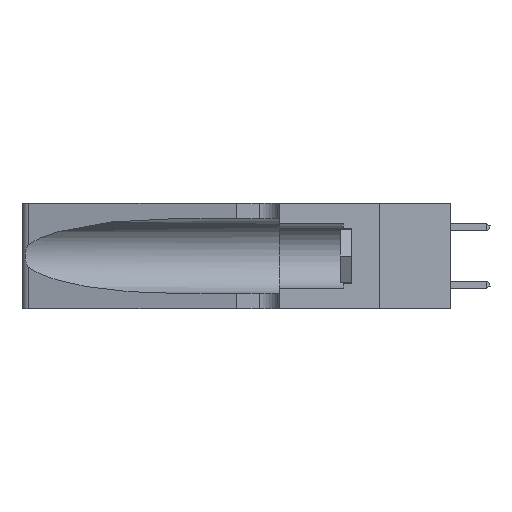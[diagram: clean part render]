
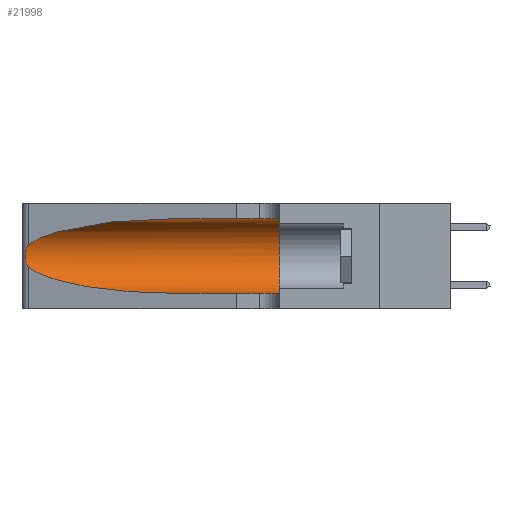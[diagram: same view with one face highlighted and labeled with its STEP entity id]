
A CAD part, left-side view. The second image highlights one B-rep face of the part: STEP entity #21998.
In plain terms, the highlighted cylindrical face has radius 3.308 mm (diameter 6.617 mm), a partial arc.
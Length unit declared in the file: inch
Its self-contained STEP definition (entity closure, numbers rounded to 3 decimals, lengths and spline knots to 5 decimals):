
#524 = CARTESIAN_POINT ( 'NONE',  ( 0.25487, 1.22718, 0.14631 ) ) ;
#641 = VERTEX_POINT ( 'NONE', #1984 ) ;
#919 = ORIENTED_EDGE ( 'NONE', *, *, #20815, .T. ) ;
#1160 = DIRECTION ( 'NONE',  ( 0., -1., 0. ) ) ;
#1449 = CYLINDRICAL_SURFACE ( 'NONE', #28516, 0.13025 ) ;
#1646 = VERTEX_POINT ( 'NONE', #9992 ) ;
#1953 = CARTESIAN_POINT ( 'NONE',  ( 0.25787, 1.23484, 0.2124 ) ) ;
#1984 = CARTESIAN_POINT ( 'NONE',  ( 0.1305, 0.72297, 0.31525 ) ) ;
#2099 = LINE ( 'NONE', #20987, #19862 ) ;
#2446 =( BOUNDED_CURVE ( )  B_SPLINE_CURVE ( 3, ( #29712, #20553, #8899, #18392 ),
 .UNSPECIFIED., .F., .F. ) 
 B_SPLINE_CURVE_WITH_KNOTS ( ( 4, 4 ),
 ( 1.5708, 2.84003 ),
 .UNSPECIFIED. ) 
 CURVE ( )  GEOMETRIC_REPRESENTATION_ITEM ( )  RATIONAL_B_SPLINE_CURVE ( ( 1., 0.87, 0.87, 1. ) ) 
 REPRESENTATION_ITEM ( '' )  );
#2768 = ORIENTED_EDGE ( 'NONE', *, *, #12227, .T. ) ;
#3309 = EDGE_CURVE ( 'NONE', #641, #1646, #25757, .T. ) ;
#3531 = CARTESIAN_POINT ( 'NONE',  ( 0.26075, 1.23896, 0.178 ) ) ;
#3865 = EDGE_CURVE ( 'NONE', #14556, #19030, #2099, .T. ) ;
#4131 = CARTESIAN_POINT ( 'NONE',  ( 0.25487, 1.22718, 0.14631 ) ) ;
#4221 = ORIENTED_EDGE ( 'NONE', *, *, #3309, .F. ) ;
#5302 = DIRECTION ( 'NONE',  ( 0., -1., 0. ) ) ;
#6467 = CARTESIAN_POINT ( 'NONE',  ( 0.25487, 1.22718, 0.14631 ) ) ;
#8374 = CARTESIAN_POINT ( 'NONE',  ( 0.25856, 1.23593, 0.16098 ) ) ;
#8885 = CARTESIAN_POINT ( 'NONE',  ( 0.25789, 1.23486, 0.15765 ) ) ;
#8899 = CARTESIAN_POINT ( 'NONE',  ( 0.2373, 1.15595, 0.28018 ) ) ;
#9102 = CARTESIAN_POINT ( 'NONE',  ( 0.26017, 1.23833, 0.17102 ) ) ;
#9992 = CARTESIAN_POINT ( 'NONE',  ( 0.1305, 0.35, 0.31525 ) ) ;
#10000 = CARTESIAN_POINT ( 'NONE',  ( 0.2373, 1.15595, 0.08982 ) ) ;
#10235 = B_SPLINE_CURVE_WITH_KNOTS ( 'NONE', 3,
 ( #23210, #20645, #24772, #1953, #27136, #25475, #23007, #3531, #9102, #8374, #8885, #20744, #20036, #4131 ),
 .UNSPECIFIED., .F., .F.,
 ( 4, 2, 2, 2, 2, 2, 4 ),
 ( 0., 0.00027, 0.00053, 0.00107, 0.0016, 0.00187, 0.00214 ),
 .UNSPECIFIED. ) ;
#11833 = ORIENTED_EDGE ( 'NONE', *, *, #3865, .T. ) ;
#12227 = EDGE_CURVE ( 'NONE', #22689, #14556, #13000, .T. ) ;
#13000 =( BOUNDED_CURVE ( )  B_SPLINE_CURVE ( 3, ( #524, #10000, #17386, #19578 ),
 .UNSPECIFIED., .F., .T. ) 
 B_SPLINE_CURVE_WITH_KNOTS ( ( 4, 4 ),
 ( 3.44316, 4.71239 ),
 .UNSPECIFIED. ) 
 CURVE ( )  GEOMETRIC_REPRESENTATION_ITEM ( )  RATIONAL_B_SPLINE_CURVE ( ( 1., 0.87, 0.87, 1. ) ) 
 REPRESENTATION_ITEM ( '' )  );
#13877 = EDGE_LOOP ( 'NONE', ( #28244, #919, #2768, #11833, #23106, #4221 ) ) ;
#14210 = EDGE_CURVE ( 'NONE', #641, #27275, #2446, .T. ) ;
#14556 = VERTEX_POINT ( 'NONE', #19638 ) ;
#15070 = CARTESIAN_POINT ( 'NONE',  ( 0.1305, 0.35, 0.185 ) ) ;
#15837 = CARTESIAN_POINT ( 'NONE',  ( 0.1305, 0.35, 0.05475 ) ) ;
#15981 = CARTESIAN_POINT ( 'NONE',  ( 0.25487, 1.22718, 0.22369 ) ) ;
#16174 = VECTOR ( 'NONE', #5302, 39.37008 ) ;
#16952 = CARTESIAN_POINT ( 'NONE',  ( 0.1305, 1.61858, 0.31525 ) ) ;
#17386 = CARTESIAN_POINT ( 'NONE',  ( 0.18966, 0.96281, 0.05475 ) ) ;
#17399 = DIRECTION ( 'NONE',  ( 0., 0., -1. ) ) ;
#17624 = AXIS2_PLACEMENT_3D ( 'NONE', #15070, #19726, #22057 ) ;
#18392 = CARTESIAN_POINT ( 'NONE',  ( 0.25487, 1.22718, 0.22369 ) ) ;
#19030 = VERTEX_POINT ( 'NONE', #15837 ) ;
#19578 = CARTESIAN_POINT ( 'NONE',  ( 0.1305, 0.72297, 0.05475 ) ) ;
#19638 = CARTESIAN_POINT ( 'NONE',  ( 0.1305, 0.72297, 0.05475 ) ) ;
#19726 = DIRECTION ( 'NONE',  ( 0., 1., 0. ) ) ;
#19862 = VECTOR ( 'NONE', #25723, 39.37008 ) ;
#19982 = CARTESIAN_POINT ( 'NONE',  ( 0.1305, 1.61858, 0.185 ) ) ;
#20036 = CARTESIAN_POINT ( 'NONE',  ( 0.25555, 1.22993, 0.14849 ) ) ;
#20319 = FACE_OUTER_BOUND ( 'NONE', #13877, .T. ) ;
#20553 = CARTESIAN_POINT ( 'NONE',  ( 0.18966, 0.96281, 0.31525 ) ) ;
#20645 = CARTESIAN_POINT ( 'NONE',  ( 0.25555, 1.22994, 0.2215 ) ) ;
#20744 = CARTESIAN_POINT ( 'NONE',  ( 0.25639, 1.23186, 0.15144 ) ) ;
#20815 = EDGE_CURVE ( 'NONE', #27275, #22689, #10235, .T. ) ;
#20987 = CARTESIAN_POINT ( 'NONE',  ( 0.1305, 1.61858, 0.05475 ) ) ;
#21752 = CIRCLE ( 'NONE', #17624, 0.13025 ) ;
#21998 = ADVANCED_FACE ( 'NONE', ( #20319 ), #1449, .F. ) ;
#22057 = DIRECTION ( 'NONE',  ( 0., 0., 1. ) ) ;
#22689 = VERTEX_POINT ( 'NONE', #6467 ) ;
#23007 = CARTESIAN_POINT ( 'NONE',  ( 0.26075, 1.23896, 0.19203 ) ) ;
#23106 = ORIENTED_EDGE ( 'NONE', *, *, #30399, .F. ) ;
#23210 = CARTESIAN_POINT ( 'NONE',  ( 0.25487, 1.22718, 0.22369 ) ) ;
#24772 = CARTESIAN_POINT ( 'NONE',  ( 0.25639, 1.23184, 0.21858 ) ) ;
#25475 = CARTESIAN_POINT ( 'NONE',  ( 0.26018, 1.23835, 0.19895 ) ) ;
#25723 = DIRECTION ( 'NONE',  ( 0., -1., 0. ) ) ;
#25757 = LINE ( 'NONE', #16952, #16174 ) ;
#27136 = CARTESIAN_POINT ( 'NONE',  ( 0.25854, 1.2359, 0.20912 ) ) ;
#27275 = VERTEX_POINT ( 'NONE', #15981 ) ;
#28244 = ORIENTED_EDGE ( 'NONE', *, *, #14210, .T. ) ;
#28516 = AXIS2_PLACEMENT_3D ( 'NONE', #19982, #1160, #17399 ) ;
#29712 = CARTESIAN_POINT ( 'NONE',  ( 0.1305, 0.72297, 0.31525 ) ) ;
#30399 = EDGE_CURVE ( 'NONE', #1646, #19030, #21752, .T. ) ;
